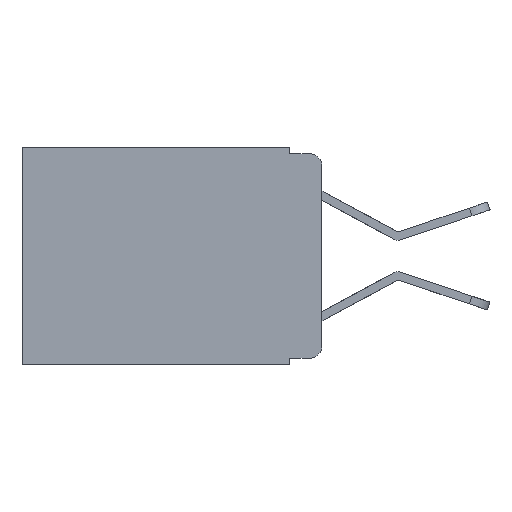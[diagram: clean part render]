
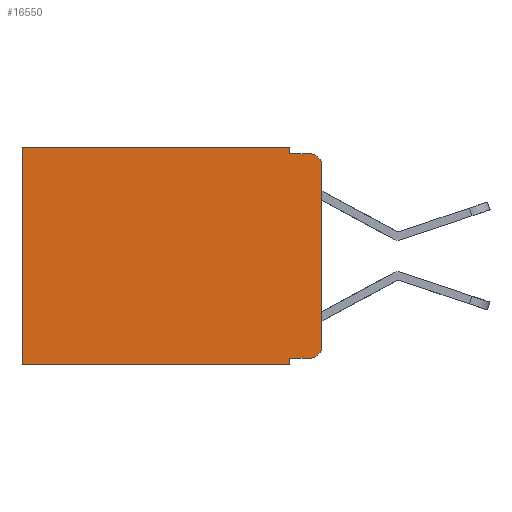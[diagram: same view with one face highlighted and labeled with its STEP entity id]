
A CAD part, left-side view. The second image highlights one B-rep face of the part: STEP entity #16550.
In plain terms, the highlighted planar face has unit normal (-1, 0, 0).
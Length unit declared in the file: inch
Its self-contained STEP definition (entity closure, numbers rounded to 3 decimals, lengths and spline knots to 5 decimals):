
#300 = CARTESIAN_POINT ( 'NONE',  ( 0.298, 0., 0. ) ) ;
#1395 = CARTESIAN_POINT ( 'NONE',  ( 0.298, 0.051, -0.333 ) ) ;
#1498 = CIRCLE ( 'NONE', #10299, 0.02 ) ;
#1501 = CARTESIAN_POINT ( 'NONE',  ( 0.298, 0.051, 0. ) ) ;
#1969 = LINE ( 'NONE', #9206, #3257 ) ;
#2279 = ORIENTED_EDGE ( 'NONE', *, *, #6599, .T. ) ;
#2305 = AXIS2_PLACEMENT_3D ( 'NONE', #15085, #3487, #16918 ) ;
#2383 = CARTESIAN_POINT ( 'NONE',  ( 0.298, 0.473, -0.343 ) ) ;
#3018 = DIRECTION ( 'NONE',  ( 0., 0., -1. ) ) ;
#3250 = CARTESIAN_POINT ( 'NONE',  ( 0.298, 0.02, -0.333 ) ) ;
#3257 = VECTOR ( 'NONE', #20257, 39.37008 ) ;
#3487 = DIRECTION ( 'NONE',  ( -1., 0., 0. ) ) ;
#3959 = DIRECTION ( 'NONE',  ( -1., 0., 0. ) ) ;
#4039 = FACE_OUTER_BOUND ( 'NONE', #15831, .T. ) ;
#4113 = LINE ( 'NONE', #1501, #19777 ) ;
#4695 = CARTESIAN_POINT ( 'NONE',  ( 0.298, 0.473, 0. ) ) ;
#4746 = VERTEX_POINT ( 'NONE', #19639 ) ;
#5942 = DIRECTION ( 'NONE',  ( 0., -1., 0. ) ) ;
#6260 = EDGE_CURVE ( 'NONE', #11189, #23509, #13828, .T. ) ;
#6526 = EDGE_CURVE ( 'NONE', #13795, #4746, #15531, .T. ) ;
#6534 = EDGE_CURVE ( 'NONE', #24171, #13795, #24516, .T. ) ;
#6566 = EDGE_CURVE ( 'NONE', #24171, #12805, #4113, .T. ) ;
#6599 = EDGE_CURVE ( 'NONE', #23509, #7212, #22867, .T. ) ;
#6604 = EDGE_CURVE ( 'NONE', #11189, #15438, #13180, .T. ) ;
#6644 = EDGE_CURVE ( 'NONE', #15438, #21285, #7621, .T. ) ;
#6652 = EDGE_CURVE ( 'NONE', #13862, #21285, #1498, .T. ) ;
#6721 = EDGE_CURVE ( 'NONE', #13862, #4746, #19496, .T. ) ;
#7212 = VERTEX_POINT ( 'NONE', #2383 ) ;
#7621 = LINE ( 'NONE', #24354, #21202 ) ;
#8213 = VECTOR ( 'NONE', #20626, 39.37008 ) ;
#8630 = ORIENTED_EDGE ( 'NONE', *, *, #6534, .T. ) ;
#9206 = CARTESIAN_POINT ( 'NONE',  ( 0.298, 0., -0.343 ) ) ;
#9480 = ORIENTED_EDGE ( 'NONE', *, *, #6652, .T. ) ;
#10299 = AXIS2_PLACEMENT_3D ( 'NONE', #15474, #3959, #17323 ) ;
#10644 = CARTESIAN_POINT ( 'NONE',  ( 0.298, 0.051, -0.343 ) ) ;
#10956 = EDGE_CURVE ( 'NONE', #12805, #7212, #1969, .T. ) ;
#11189 = VERTEX_POINT ( 'NONE', #17780 ) ;
#12127 = ORIENTED_EDGE ( 'NONE', *, *, #10956, .F. ) ;
#12805 = VERTEX_POINT ( 'NONE', #10644 ) ;
#13180 = LINE ( 'NONE', #20703, #22302 ) ;
#13207 = VECTOR ( 'NONE', #17820, 39.37008 ) ;
#13273 = DIRECTION ( 'NONE',  ( 0., 0., -1. ) ) ;
#13301 = ORIENTED_EDGE ( 'NONE', *, *, #6604, .F. ) ;
#13795 = VERTEX_POINT ( 'NONE', #3250 ) ;
#13828 = LINE ( 'NONE', #300, #13207 ) ;
#13862 = VERTEX_POINT ( 'NONE', #20498 ) ;
#14686 = DIRECTION ( 'NONE',  ( 1., 0., 0. ) ) ;
#15068 = ORIENTED_EDGE ( 'NONE', *, *, #6721, .F. ) ;
#15085 = CARTESIAN_POINT ( 'NONE',  ( 0.298, 0.02, -0.313 ) ) ;
#15438 = VERTEX_POINT ( 'NONE', #19238 ) ;
#15474 = CARTESIAN_POINT ( 'NONE',  ( 0.298, 0.02, -0.03 ) ) ;
#15531 = CIRCLE ( 'NONE', #2305, 0.02 ) ;
#15831 = EDGE_LOOP ( 'NONE', ( #15068, #9480, #23518, #13301, #22398, #2279, #12127, #23802, #8630, #22701 ) ) ;
#15876 = CARTESIAN_POINT ( 'NONE',  ( 0.298, 0.02, -0.01 ) ) ;
#16049 = AXIS2_PLACEMENT_3D ( 'NONE', #21730, #14686, #3018 ) ;
#16550 = ADVANCED_FACE ( 'NONE', ( #4039 ), #18243, .F. ) ;
#16918 = DIRECTION ( 'NONE',  ( 0., 0., -1. ) ) ;
#17323 = DIRECTION ( 'NONE',  ( 0., 0., -1. ) ) ;
#17780 = CARTESIAN_POINT ( 'NONE',  ( 0.298, 0.051, 0. ) ) ;
#17820 = DIRECTION ( 'NONE',  ( 0., 1., 0. ) ) ;
#18243 = PLANE ( 'NONE',  #16049 ) ;
#18720 = DIRECTION ( 'NONE',  ( 0., -1., 0. ) ) ;
#19225 = VECTOR ( 'NONE', #18720, 39.37008 ) ;
#19238 = CARTESIAN_POINT ( 'NONE',  ( 0.298, 0.051, -0.01 ) ) ;
#19283 = CARTESIAN_POINT ( 'NONE',  ( 0.298, 0., 0. ) ) ;
#19496 = LINE ( 'NONE', #19283, #23685 ) ;
#19504 = CARTESIAN_POINT ( 'NONE',  ( 0.298, 0.051, -0.333 ) ) ;
#19639 = CARTESIAN_POINT ( 'NONE',  ( 0.298, 0., -0.313 ) ) ;
#19777 = VECTOR ( 'NONE', #13273, 39.37008 ) ;
#20257 = DIRECTION ( 'NONE',  ( 0., 1., 0. ) ) ;
#20498 = CARTESIAN_POINT ( 'NONE',  ( 0.298, 0., -0.03 ) ) ;
#20626 = DIRECTION ( 'NONE',  ( 0., 0., -1. ) ) ;
#20703 = CARTESIAN_POINT ( 'NONE',  ( 0.298, 0.051, 0. ) ) ;
#21101 = DIRECTION ( 'NONE',  ( 0., 0., -1. ) ) ;
#21202 = VECTOR ( 'NONE', #5942, 39.37008 ) ;
#21285 = VERTEX_POINT ( 'NONE', #15876 ) ;
#21730 = CARTESIAN_POINT ( 'NONE',  ( 0.298, 0., 0. ) ) ;
#22302 = VECTOR ( 'NONE', #22412, 39.37008 ) ;
#22398 = ORIENTED_EDGE ( 'NONE', *, *, #6260, .T. ) ;
#22412 = DIRECTION ( 'NONE',  ( 0., 0., -1. ) ) ;
#22701 = ORIENTED_EDGE ( 'NONE', *, *, #6526, .T. ) ;
#22867 = LINE ( 'NONE', #24203, #8213 ) ;
#23509 = VERTEX_POINT ( 'NONE', #4695 ) ;
#23518 = ORIENTED_EDGE ( 'NONE', *, *, #6644, .F. ) ;
#23685 = VECTOR ( 'NONE', #21101, 39.37008 ) ;
#23802 = ORIENTED_EDGE ( 'NONE', *, *, #6566, .F. ) ;
#24171 = VERTEX_POINT ( 'NONE', #19504 ) ;
#24203 = CARTESIAN_POINT ( 'NONE',  ( 0.298, 0.473, 0. ) ) ;
#24354 = CARTESIAN_POINT ( 'NONE',  ( 0.298, 0.051, -0.01 ) ) ;
#24516 = LINE ( 'NONE', #1395, #19225 ) ;
